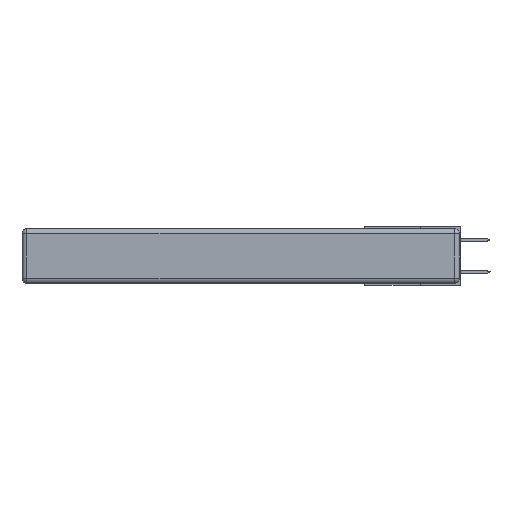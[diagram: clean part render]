
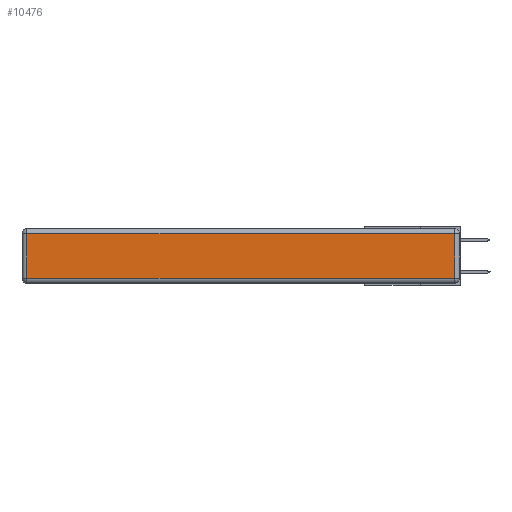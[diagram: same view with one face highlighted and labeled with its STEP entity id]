
A CAD part, left-side view. The second image highlights one B-rep face of the part: STEP entity #10476.
In plain terms, the highlighted planar face has unit normal (-1, 0, 0).
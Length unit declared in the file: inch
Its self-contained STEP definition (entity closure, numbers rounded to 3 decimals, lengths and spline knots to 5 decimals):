
#207 = CARTESIAN_POINT ( 'NONE',  ( 0., 0., -0.313 ) ) ;
#320 = ORIENTED_EDGE ( 'NONE', *, *, #7492, .T. ) ;
#359 = VERTEX_POINT ( 'NONE', #7368 ) ;
#749 = AXIS2_PLACEMENT_3D ( 'NONE', #11840, #5632, #4509 ) ;
#1229 = VECTOR ( 'NONE', #12969, 39.37008 ) ;
#1439 = ORIENTED_EDGE ( 'NONE', *, *, #2173, .T. ) ;
#2029 = VERTEX_POINT ( 'NONE', #2112 ) ;
#2112 = CARTESIAN_POINT ( 'NONE',  ( 0., 0.03, -0.313 ) ) ;
#2173 = EDGE_CURVE ( 'NONE', #359, #10366, #4477, .T. ) ;
#2288 = CARTESIAN_POINT ( 'NONE',  ( 0., 2.72, -0.343 ) ) ;
#3000 = EDGE_CURVE ( 'NONE', #2029, #359, #12761, .T. ) ;
#3033 = CARTESIAN_POINT ( 'NONE',  ( 0., 0.03, -0.343 ) ) ;
#3518 = CARTESIAN_POINT ( 'NONE',  ( 0., 2.72, -0.03 ) ) ;
#4161 = LINE ( 'NONE', #207, #7907 ) ;
#4260 = CARTESIAN_POINT ( 'NONE',  ( 0., 2.72, -0.313 ) ) ;
#4477 = LINE ( 'NONE', #10843, #1229 ) ;
#4509 = DIRECTION ( 'NONE',  ( 0., 0., 1. ) ) ;
#4527 = DIRECTION ( 'NONE',  ( 0., -1., 0. ) ) ;
#4555 = PLANE ( 'NONE',  #749 ) ;
#5632 = DIRECTION ( 'NONE',  ( -1., 0., 0. ) ) ;
#5685 = EDGE_CURVE ( 'NONE', #10366, #12410, #10558, .T. ) ;
#7368 = CARTESIAN_POINT ( 'NONE',  ( 0., 0.03, -0.03 ) ) ;
#7492 = EDGE_CURVE ( 'NONE', #12410, #2029, #4161, .T. ) ;
#7907 = VECTOR ( 'NONE', #4527, 39.37008 ) ;
#8119 = ORIENTED_EDGE ( 'NONE', *, *, #3000, .T. ) ;
#8528 = DIRECTION ( 'NONE',  ( 0., 0., -1. ) ) ;
#9374 = EDGE_LOOP ( 'NONE', ( #320, #8119, #1439, #13414 ) ) ;
#10366 = VERTEX_POINT ( 'NONE', #3518 ) ;
#10428 = FACE_OUTER_BOUND ( 'NONE', #9374, .T. ) ;
#10466 = DIRECTION ( 'NONE',  ( 0., 0., 1. ) ) ;
#10476 = ADVANCED_FACE ( 'NONE', ( #10428 ), #4555, .T. ) ;
#10558 = LINE ( 'NONE', #2288, #11203 ) ;
#10843 = CARTESIAN_POINT ( 'NONE',  ( 0., 2.75, -0.03 ) ) ;
#11203 = VECTOR ( 'NONE', #8528, 39.37008 ) ;
#11840 = CARTESIAN_POINT ( 'NONE',  ( 0., 0., -0.343 ) ) ;
#12269 = VECTOR ( 'NONE', #10466, 39.37008 ) ;
#12410 = VERTEX_POINT ( 'NONE', #4260 ) ;
#12761 = LINE ( 'NONE', #3033, #12269 ) ;
#12969 = DIRECTION ( 'NONE',  ( 0., 1., 0. ) ) ;
#13414 = ORIENTED_EDGE ( 'NONE', *, *, #5685, .T. ) ;
